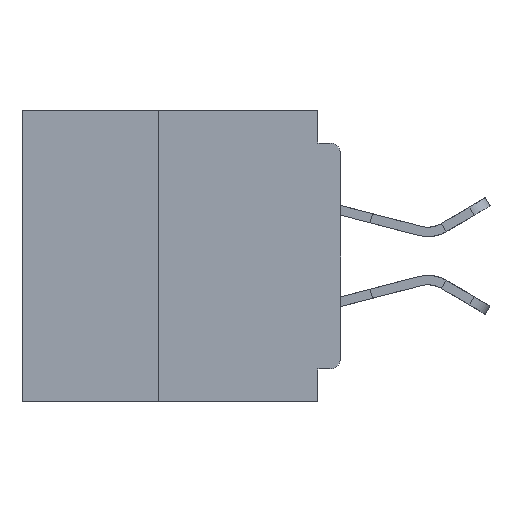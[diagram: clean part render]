
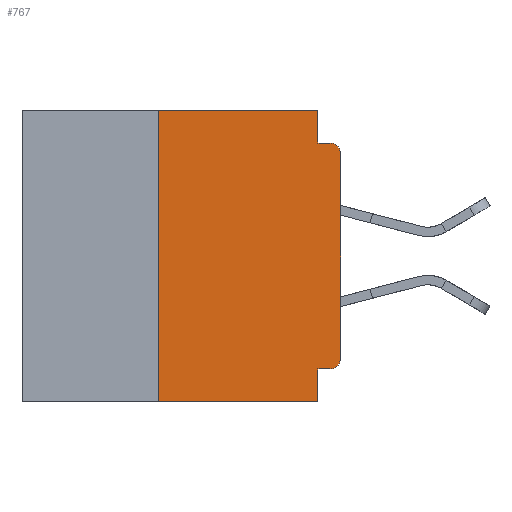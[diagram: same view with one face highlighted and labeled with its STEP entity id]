
A CAD part, left-side view. The second image highlights one B-rep face of the part: STEP entity #767.
In plain terms, the highlighted planar face has unit normal (-1, 0, 0).
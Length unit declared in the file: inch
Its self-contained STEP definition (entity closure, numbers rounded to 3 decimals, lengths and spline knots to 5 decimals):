
#724 = ORIENTED_EDGE ( 'NONE', *, *, #20310, .T. ) ;
#767 = ADVANCED_FACE ( 'NONE', ( #9281 ), #6102, .F. ) ;
#1547 = VECTOR ( 'NONE', #1782, 39.37008 ) ;
#1782 = DIRECTION ( 'NONE',  ( 0., 0., -1. ) ) ;
#1911 = VERTEX_POINT ( 'NONE', #18787 ) ;
#2149 = CARTESIAN_POINT ( 'NONE',  ( 0., 0.25, 0. ) ) ;
#2189 = CARTESIAN_POINT ( 'NONE',  ( 0., 0.015, -0.06 ) ) ;
#3361 = VERTEX_POINT ( 'NONE', #13092 ) ;
#3814 = LINE ( 'NONE', #6662, #34491 ) ;
#4220 = EDGE_CURVE ( 'NONE', #7376, #30022, #21029, .T. ) ;
#4246 = CARTESIAN_POINT ( 'NONE',  ( 0., 0.015, -0.34 ) ) ;
#4683 = CARTESIAN_POINT ( 'NONE',  ( 0., 0., -0.355 ) ) ;
#5079 = CARTESIAN_POINT ( 'NONE',  ( 0., 0., 0. ) ) ;
#5081 = VECTOR ( 'NONE', #23029, 39.37008 ) ;
#5257 = VECTOR ( 'NONE', #31236, 39.37008 ) ;
#5316 = DIRECTION ( 'NONE',  ( 0., 0., -1. ) ) ;
#5771 = DIRECTION ( 'NONE',  ( 1., 0., 0. ) ) ;
#5857 = DIRECTION ( 'NONE',  ( 0., 0., -1. ) ) ;
#5957 = CARTESIAN_POINT ( 'NONE',  ( 0., 0.437, 0. ) ) ;
#6102 = PLANE ( 'NONE',  #28918 ) ;
#6178 = ORIENTED_EDGE ( 'NONE', *, *, #28022, .F. ) ;
#6227 = DIRECTION ( 'NONE',  ( 0., -1., 0. ) ) ;
#6662 = CARTESIAN_POINT ( 'NONE',  ( 0., 0.25, -0.4 ) ) ;
#7016 = VECTOR ( 'NONE', #6227, 39.37008 ) ;
#7020 = CARTESIAN_POINT ( 'NONE',  ( 0., 0.015, -0.355 ) ) ;
#7344 = DIRECTION ( 'NONE',  ( 0., 0., -1. ) ) ;
#7376 = VERTEX_POINT ( 'NONE', #12456 ) ;
#7533 = VERTEX_POINT ( 'NONE', #7020 ) ;
#7855 = CARTESIAN_POINT ( 'NONE',  ( 0., 0.25, -0.4 ) ) ;
#8563 = CARTESIAN_POINT ( 'NONE',  ( 0., 0.031, 0. ) ) ;
#8841 = VERTEX_POINT ( 'NONE', #9700 ) ;
#9281 = FACE_OUTER_BOUND ( 'NONE', #10013, .T. ) ;
#9700 = CARTESIAN_POINT ( 'NONE',  ( 0., 0.031, -0.4 ) ) ;
#10013 = EDGE_LOOP ( 'NONE', ( #724, #24090, #16787, #17262, #10841, #27716, #35767, #6178, #36083, #28686 ) ) ;
#10841 = ORIENTED_EDGE ( 'NONE', *, *, #14924, .F. ) ;
#11067 = CARTESIAN_POINT ( 'NONE',  ( 0., 0.031, -0.4 ) ) ;
#12410 = CIRCLE ( 'NONE', #35600, 0.015 ) ;
#12456 = CARTESIAN_POINT ( 'NONE',  ( 0., 0.031, -0.045 ) ) ;
#13092 = CARTESIAN_POINT ( 'NONE',  ( 0., 0.031, -0.355 ) ) ;
#14924 = EDGE_CURVE ( 'NONE', #15141, #16516, #21230, .T. ) ;
#15141 = VERTEX_POINT ( 'NONE', #2149 ) ;
#16516 = VERTEX_POINT ( 'NONE', #24516 ) ;
#16787 = ORIENTED_EDGE ( 'NONE', *, *, #4220, .F. ) ;
#17105 = EDGE_CURVE ( 'NONE', #7533, #1911, #34577, .T. ) ;
#17262 = ORIENTED_EDGE ( 'NONE', *, *, #37617, .F. ) ;
#17669 = LINE ( 'NONE', #11067, #1547 ) ;
#18582 = VERTEX_POINT ( 'NONE', #32602 ) ;
#18787 = CARTESIAN_POINT ( 'NONE',  ( 0., 0., -0.34 ) ) ;
#20310 = EDGE_CURVE ( 'NONE', #1911, #18582, #29355, .T. ) ;
#20949 = LINE ( 'NONE', #4683, #37363 ) ;
#21029 = LINE ( 'NONE', #21325, #5081 ) ;
#21230 = LINE ( 'NONE', #28339, #5257 ) ;
#21325 = CARTESIAN_POINT ( 'NONE',  ( 0., 0., -0.045 ) ) ;
#21458 = DIRECTION ( 'NONE',  ( 0., 0., 1. ) ) ;
#22013 = LINE ( 'NONE', #27176, #7016 ) ;
#23029 = DIRECTION ( 'NONE',  ( 0., -1., 0. ) ) ;
#23106 = EDGE_CURVE ( 'NONE', #18582, #30022, #12410, .T. ) ;
#23340 = DIRECTION ( 'NONE',  ( -1., 0., 0. ) ) ;
#23929 = VECTOR ( 'NONE', #26560, 39.37008 ) ;
#24090 = ORIENTED_EDGE ( 'NONE', *, *, #23106, .T. ) ;
#24516 = CARTESIAN_POINT ( 'NONE',  ( 0., 0.031, 0. ) ) ;
#25258 = DIRECTION ( 'NONE',  ( -1., 0., 0. ) ) ;
#25708 = DIRECTION ( 'NONE',  ( 0., 1., 0. ) ) ;
#26087 = DIRECTION ( 'NONE',  ( 0., 0., 1. ) ) ;
#26560 = DIRECTION ( 'NONE',  ( 0., 0., -1. ) ) ;
#27176 = CARTESIAN_POINT ( 'NONE',  ( 0., 0.437, -0.4 ) ) ;
#27716 = ORIENTED_EDGE ( 'NONE', *, *, #33806, .F. ) ;
#28022 = EDGE_CURVE ( 'NONE', #3361, #8841, #17669, .T. ) ;
#28339 = CARTESIAN_POINT ( 'NONE',  ( 0., 0.437, 0. ) ) ;
#28456 = VECTOR ( 'NONE', #26087, 39.37008 ) ;
#28547 = VERTEX_POINT ( 'NONE', #7855 ) ;
#28686 = ORIENTED_EDGE ( 'NONE', *, *, #17105, .T. ) ;
#28918 = AXIS2_PLACEMENT_3D ( 'NONE', #5957, #5771, #5857 ) ;
#29355 = LINE ( 'NONE', #5079, #28456 ) ;
#29954 = EDGE_CURVE ( 'NONE', #28547, #8841, #22013, .T. ) ;
#30022 = VERTEX_POINT ( 'NONE', #33206 ) ;
#30952 = EDGE_CURVE ( 'NONE', #7533, #3361, #20949, .T. ) ;
#31236 = DIRECTION ( 'NONE',  ( 0., -1., 0. ) ) ;
#32578 = LINE ( 'NONE', #8563, #23929 ) ;
#32602 = CARTESIAN_POINT ( 'NONE',  ( 0., 0., -0.06 ) ) ;
#33206 = CARTESIAN_POINT ( 'NONE',  ( 0., 0.015, -0.045 ) ) ;
#33806 = EDGE_CURVE ( 'NONE', #28547, #15141, #3814, .T. ) ;
#34305 = AXIS2_PLACEMENT_3D ( 'NONE', #4246, #25258, #7344 ) ;
#34491 = VECTOR ( 'NONE', #21458, 39.37008 ) ;
#34577 = CIRCLE ( 'NONE', #34305, 0.015 ) ;
#35600 = AXIS2_PLACEMENT_3D ( 'NONE', #2189, #23340, #5316 ) ;
#35767 = ORIENTED_EDGE ( 'NONE', *, *, #29954, .T. ) ;
#36083 = ORIENTED_EDGE ( 'NONE', *, *, #30952, .F. ) ;
#37363 = VECTOR ( 'NONE', #25708, 39.37008 ) ;
#37617 = EDGE_CURVE ( 'NONE', #16516, #7376, #32578, .T. ) ;
